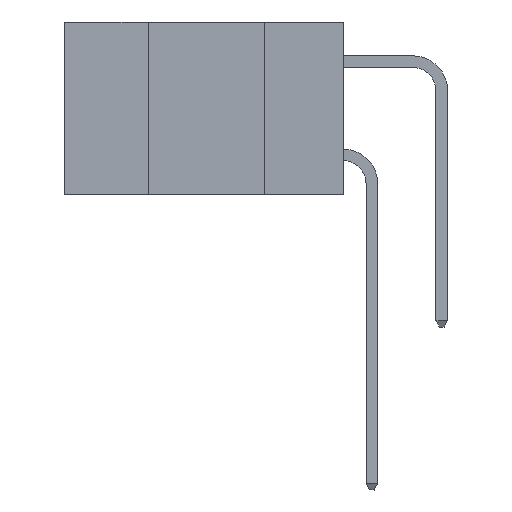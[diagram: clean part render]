
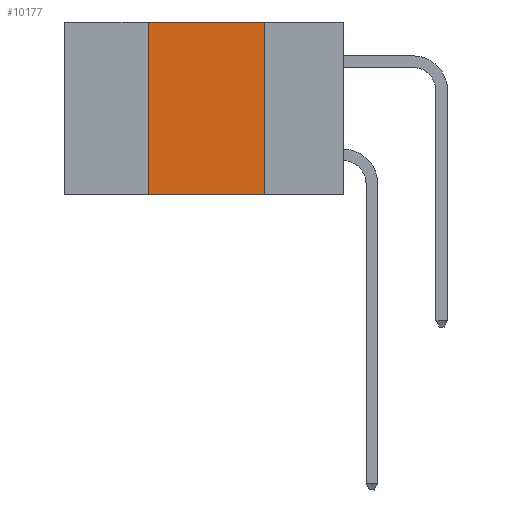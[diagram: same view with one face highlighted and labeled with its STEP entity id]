
A CAD part, left-side view. The second image highlights one B-rep face of the part: STEP entity #10177.
In plain terms, the highlighted planar face has unit normal (-1, 0, 0).
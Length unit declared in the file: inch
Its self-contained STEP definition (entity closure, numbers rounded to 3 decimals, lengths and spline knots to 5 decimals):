
#44 = DIRECTION ( 'NONE',  ( 0., 0., -1. ) ) ;
#420 = LINE ( 'NONE', #2852, #16758 ) ;
#1042 = PLANE ( 'NONE',  #6513 ) ;
#1123 = CARTESIAN_POINT ( 'NONE',  ( 0., 0.6, 0. ) ) ;
#1705 = DIRECTION ( 'NONE',  ( 0., -1., 0. ) ) ;
#1744 = EDGE_CURVE ( 'NONE', #1997, #2098, #420, .T. ) ;
#1997 = VERTEX_POINT ( 'NONE', #10179 ) ;
#2098 = VERTEX_POINT ( 'NONE', #12741 ) ;
#2591 = ORIENTED_EDGE ( 'NONE', *, *, #16231, .T. ) ;
#2731 = VERTEX_POINT ( 'NONE', #12427 ) ;
#2852 = CARTESIAN_POINT ( 'NONE',  ( 0., 0.17, -0.37 ) ) ;
#3661 = VERTEX_POINT ( 'NONE', #16644 ) ;
#3849 = VECTOR ( 'NONE', #7785, 39.37008 ) ;
#3935 = LINE ( 'NONE', #7711, #3849 ) ;
#5006 = LINE ( 'NONE', #10211, #11209 ) ;
#6513 = AXIS2_PLACEMENT_3D ( 'NONE', #1123, #12966, #44 ) ;
#6610 = DIRECTION ( 'NONE',  ( 0., -1., 0. ) ) ;
#6732 = ORIENTED_EDGE ( 'NONE', *, *, #15699, .F. ) ;
#7711 = CARTESIAN_POINT ( 'NONE',  ( 0., 0.42, -0.37 ) ) ;
#7785 = DIRECTION ( 'NONE',  ( 0., 0., 1. ) ) ;
#8777 = FACE_OUTER_BOUND ( 'NONE', #16134, .T. ) ;
#10177 = ADVANCED_FACE ( 'NONE', ( #8777 ), #1042, .F. ) ;
#10179 = CARTESIAN_POINT ( 'NONE',  ( 0., 0.17, 0. ) ) ;
#10211 = CARTESIAN_POINT ( 'NONE',  ( 0., 0.6, 0. ) ) ;
#11209 = VECTOR ( 'NONE', #6610, 39.37008 ) ;
#11812 = DIRECTION ( 'NONE',  ( 0., 0., -1. ) ) ;
#12188 = CARTESIAN_POINT ( 'NONE',  ( 0., 0.6, -0.37 ) ) ;
#12427 = CARTESIAN_POINT ( 'NONE',  ( 0., 0.42, -0.37 ) ) ;
#12741 = CARTESIAN_POINT ( 'NONE',  ( 0., 0.17, -0.37 ) ) ;
#12966 = DIRECTION ( 'NONE',  ( 1., 0., 0. ) ) ;
#13427 = VECTOR ( 'NONE', #1705, 39.37008 ) ;
#13806 = ORIENTED_EDGE ( 'NONE', *, *, #15296, .F. ) ;
#14415 = LINE ( 'NONE', #12188, #13427 ) ;
#15296 = EDGE_CURVE ( 'NONE', #3661, #1997, #5006, .T. ) ;
#15599 = ORIENTED_EDGE ( 'NONE', *, *, #1744, .F. ) ;
#15699 = EDGE_CURVE ( 'NONE', #2731, #3661, #3935, .T. ) ;
#16134 = EDGE_LOOP ( 'NONE', ( #15599, #13806, #6732, #2591 ) ) ;
#16231 = EDGE_CURVE ( 'NONE', #2731, #2098, #14415, .T. ) ;
#16644 = CARTESIAN_POINT ( 'NONE',  ( 0., 0.42, 0. ) ) ;
#16758 = VECTOR ( 'NONE', #11812, 39.37008 ) ;
